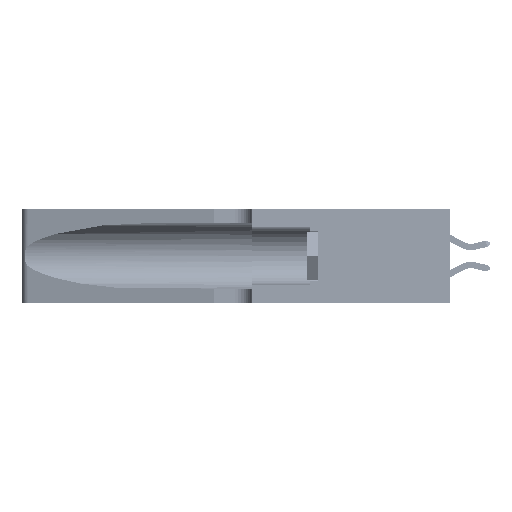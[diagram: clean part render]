
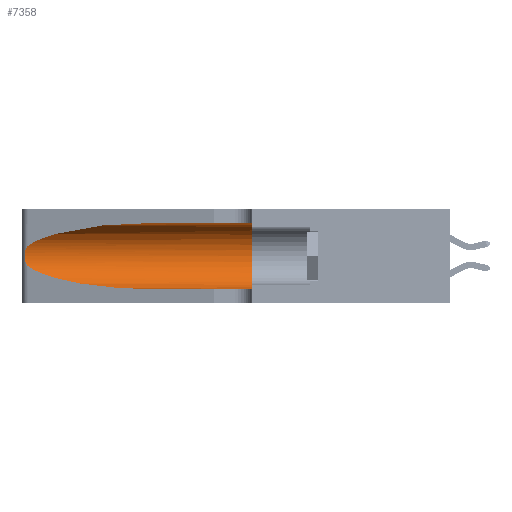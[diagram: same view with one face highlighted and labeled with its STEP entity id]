
A CAD part, left-side view. The second image highlights one B-rep face of the part: STEP entity #7358.
In plain terms, the highlighted cylindrical face has radius 3.308 mm (diameter 6.617 mm), a partial arc.
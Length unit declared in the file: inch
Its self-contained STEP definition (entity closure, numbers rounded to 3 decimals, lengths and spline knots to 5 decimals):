
#218 = CARTESIAN_POINT ( 'NONE',  ( 0.1305, 0.72297, 0.05475 ) ) ;
#1069 = CARTESIAN_POINT ( 'NONE',  ( 0.25856, 1.23593, 0.16098 ) ) ;
#3217 = VERTEX_POINT ( 'NONE', #218 ) ;
#4725 = CARTESIAN_POINT ( 'NONE',  ( 0.25639, 1.23184, 0.21858 ) ) ;
#4882 = CARTESIAN_POINT ( 'NONE',  ( 0.25639, 1.23186, 0.15144 ) ) ;
#6734 = CARTESIAN_POINT ( 'NONE',  ( 0.25487, 1.22718, 0.14631 ) ) ;
#7358 = ADVANCED_FACE ( 'NONE', ( #24437 ), #42363, .F. ) ;
#8297 = AXIS2_PLACEMENT_3D ( 'NONE', #38292, #16739, #41897 ) ;
#8386 = CARTESIAN_POINT ( 'NONE',  ( 0.1305, 0.72297, 0.31525 ) ) ;
#8450 = CARTESIAN_POINT ( 'NONE',  ( 0.1305, 1.61858, 0.185 ) ) ;
#8636 = CARTESIAN_POINT ( 'NONE',  ( 0.25487, 1.22718, 0.14631 ) ) ;
#12058 = CARTESIAN_POINT ( 'NONE',  ( 0.25555, 1.22994, 0.2215 ) ) ;
#12229 = CARTESIAN_POINT ( 'NONE',  ( 0.25487, 1.22718, 0.22369 ) ) ;
#12305 = CARTESIAN_POINT ( 'NONE',  ( 0.1305, 1.61858, 0.31525 ) ) ;
#14798 = VERTEX_POINT ( 'NONE', #8386 ) ;
#14901 = ORIENTED_EDGE ( 'NONE', *, *, #41632, .T. ) ;
#15394 =( BOUNDED_CURVE ( )  B_SPLINE_CURVE ( 3, ( #6734, #35854, #17881, #43041 ),
 .UNSPECIFIED., .F., .F. ) 
 B_SPLINE_CURVE_WITH_KNOTS ( ( 4, 4 ),
 ( 3.44316, 4.71239 ),
 .UNSPECIFIED. ) 
 CURVE ( )  GEOMETRIC_REPRESENTATION_ITEM ( )  RATIONAL_B_SPLINE_CURVE ( ( 1., 0.87, 0.87, 1. ) ) 
 REPRESENTATION_ITEM ( '' )  );
#15447 = CARTESIAN_POINT ( 'NONE',  ( 0.25487, 1.22718, 0.22369 ) ) ;
#15935 = CARTESIAN_POINT ( 'NONE',  ( 0.25854, 1.2359, 0.20912 ) ) ;
#16009 = DIRECTION ( 'NONE',  ( 0., -1., 0. ) ) ;
#16739 = DIRECTION ( 'NONE',  ( 0., 1., 0. ) ) ;
#17881 = CARTESIAN_POINT ( 'NONE',  ( 0.18966, 0.96281, 0.05475 ) ) ;
#19582 = CARTESIAN_POINT ( 'NONE',  ( 0.26075, 1.23896, 0.19203 ) ) ;
#20485 = CARTESIAN_POINT ( 'NONE',  ( 0.18966, 0.96281, 0.31525 ) ) ;
#20500 = DIRECTION ( 'NONE',  ( 0., -1., 0. ) ) ;
#20638 = CARTESIAN_POINT ( 'NONE',  ( 0.2373, 1.15595, 0.28018 ) ) ;
#21106 = EDGE_LOOP ( 'NONE', ( #33429, #43935, #22413, #14901, #45347, #43039 ) ) ;
#21985 = CIRCLE ( 'NONE', #8297, 0.13025 ) ;
#22413 = ORIENTED_EDGE ( 'NONE', *, *, #23783, .T. ) ;
#23218 = CARTESIAN_POINT ( 'NONE',  ( 0.26017, 1.23833, 0.17102 ) ) ;
#23490 = EDGE_CURVE ( 'NONE', #42647, #33062, #23832, .T. ) ;
#23745 = LINE ( 'NONE', #12305, #41681 ) ;
#23783 = EDGE_CURVE ( 'NONE', #33062, #3217, #15394, .T. ) ;
#23832 = B_SPLINE_CURVE_WITH_KNOTS ( 'NONE', 3,
 ( #12229, #12058, #4725, #37473, #15935, #41078, #19582, #44739, #23218, #1069, #26852, #4882, #30450, #8636 ),
 .UNSPECIFIED., .F., .F.,
 ( 4, 2, 2, 2, 2, 2, 4 ),
 ( 0., 0.00027, 0.00053, 0.00107, 0.0016, 0.00187, 0.00214 ),
 .UNSPECIFIED. ) ;
#24437 = FACE_OUTER_BOUND ( 'NONE', #21106, .T. ) ;
#25202 = VECTOR ( 'NONE', #20500, 39.37008 ) ;
#26852 = CARTESIAN_POINT ( 'NONE',  ( 0.25789, 1.23486, 0.15765 ) ) ;
#26858 = VERTEX_POINT ( 'NONE', #41722 ) ;
#27680 = VERTEX_POINT ( 'NONE', #46272 ) ;
#30360 = EDGE_CURVE ( 'NONE', #26858, #27680, #21985, .T. ) ;
#30450 = CARTESIAN_POINT ( 'NONE',  ( 0.25555, 1.22993, 0.14849 ) ) ;
#32892 = EDGE_CURVE ( 'NONE', #14798, #26858, #23745, .T. ) ;
#33062 = VERTEX_POINT ( 'NONE', #34609 ) ;
#33429 = ORIENTED_EDGE ( 'NONE', *, *, #45467, .T. ) ;
#33621 =( BOUNDED_CURVE ( )  B_SPLINE_CURVE ( 3, ( #34967, #20485, #20638, #45807 ),
 .UNSPECIFIED., .F., .T. ) 
 B_SPLINE_CURVE_WITH_KNOTS ( ( 4, 4 ),
 ( 1.5708, 2.84003 ),
 .UNSPECIFIED. ) 
 CURVE ( )  GEOMETRIC_REPRESENTATION_ITEM ( )  RATIONAL_B_SPLINE_CURVE ( ( 1., 0.87, 0.87, 1. ) ) 
 REPRESENTATION_ITEM ( '' )  );
#33887 = DIRECTION ( 'NONE',  ( 0., 0., -1. ) ) ;
#34609 = CARTESIAN_POINT ( 'NONE',  ( 0.25487, 1.22718, 0.14631 ) ) ;
#34743 = LINE ( 'NONE', #38069, #25202 ) ;
#34967 = CARTESIAN_POINT ( 'NONE',  ( 0.1305, 0.72297, 0.31525 ) ) ;
#35854 = CARTESIAN_POINT ( 'NONE',  ( 0.2373, 1.15595, 0.08982 ) ) ;
#37473 = CARTESIAN_POINT ( 'NONE',  ( 0.25787, 1.23484, 0.2124 ) ) ;
#38069 = CARTESIAN_POINT ( 'NONE',  ( 0.1305, 1.61858, 0.05475 ) ) ;
#38292 = CARTESIAN_POINT ( 'NONE',  ( 0.1305, 0.35, 0.185 ) ) ;
#38997 = AXIS2_PLACEMENT_3D ( 'NONE', #8450, #40905, #33887 ) ;
#40905 = DIRECTION ( 'NONE',  ( 0., -1., 0. ) ) ;
#41078 = CARTESIAN_POINT ( 'NONE',  ( 0.26018, 1.23835, 0.19895 ) ) ;
#41632 = EDGE_CURVE ( 'NONE', #3217, #27680, #34743, .T. ) ;
#41681 = VECTOR ( 'NONE', #16009, 39.37008 ) ;
#41722 = CARTESIAN_POINT ( 'NONE',  ( 0.1305, 0.35, 0.31525 ) ) ;
#41897 = DIRECTION ( 'NONE',  ( 0., 0., 1. ) ) ;
#42363 = CYLINDRICAL_SURFACE ( 'NONE', #38997, 0.13025 ) ;
#42647 = VERTEX_POINT ( 'NONE', #15447 ) ;
#43039 = ORIENTED_EDGE ( 'NONE', *, *, #32892, .F. ) ;
#43041 = CARTESIAN_POINT ( 'NONE',  ( 0.1305, 0.72297, 0.05475 ) ) ;
#43935 = ORIENTED_EDGE ( 'NONE', *, *, #23490, .T. ) ;
#44739 = CARTESIAN_POINT ( 'NONE',  ( 0.26075, 1.23896, 0.178 ) ) ;
#45347 = ORIENTED_EDGE ( 'NONE', *, *, #30360, .F. ) ;
#45467 = EDGE_CURVE ( 'NONE', #14798, #42647, #33621, .T. ) ;
#45807 = CARTESIAN_POINT ( 'NONE',  ( 0.25487, 1.22718, 0.22369 ) ) ;
#46272 = CARTESIAN_POINT ( 'NONE',  ( 0.1305, 0.35, 0.05475 ) ) ;
